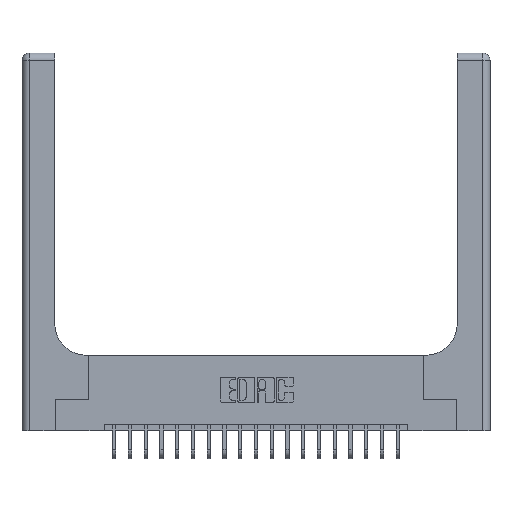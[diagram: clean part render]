
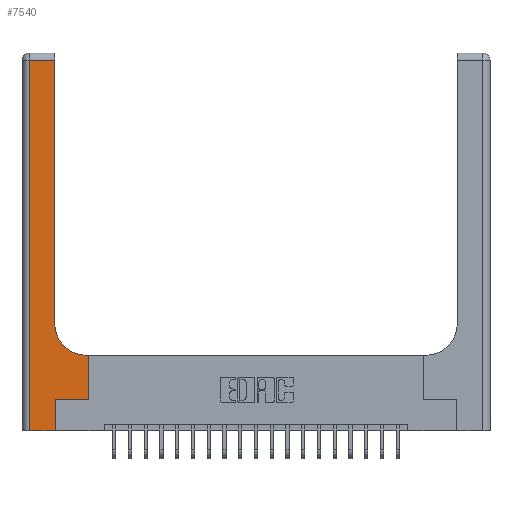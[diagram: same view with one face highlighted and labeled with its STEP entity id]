
A CAD part, top view. The second image highlights one B-rep face of the part: STEP entity #7540.
In plain terms, the highlighted planar face has unit normal (0, 0, 1).
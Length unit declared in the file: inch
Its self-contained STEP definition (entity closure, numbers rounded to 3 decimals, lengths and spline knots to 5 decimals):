
#25 = LINE ( 'NONE', #8723, #17636 ) ;
#267 = VERTEX_POINT ( 'NONE', #11001 ) ;
#465 = VERTEX_POINT ( 'NONE', #6812 ) ;
#708 = AXIS2_PLACEMENT_3D ( 'NONE', #6785, #1096, #18815 ) ;
#950 = DIRECTION ( 'NONE',  ( 0., 0., -1. ) ) ;
#1096 = DIRECTION ( 'NONE',  ( 0., 0., -1. ) ) ;
#1206 = VECTOR ( 'NONE', #18452, 39.37008 ) ;
#1271 = VERTEX_POINT ( 'NONE', #8339 ) ;
#1619 = EDGE_CURVE ( 'NONE', #19638, #19005, #4335, .T. ) ;
#1938 = ORIENTED_EDGE ( 'NONE', *, *, #16712, .T. ) ;
#2462 = CARTESIAN_POINT ( 'NONE',  ( 0.26, 2.94, 0.37 ) ) ;
#2492 = ORIENTED_EDGE ( 'NONE', *, *, #7852, .T. ) ;
#2962 = FACE_OUTER_BOUND ( 'NONE', #3066, .T. ) ;
#2971 = CARTESIAN_POINT ( 'NONE',  ( 0.26, 0.85, 0.37 ) ) ;
#3066 = EDGE_LOOP ( 'NONE', ( #18461, #1938, #12330, #13534, #17901, #19861, #5794, #11159, #2492 ) ) ;
#3070 = DIRECTION ( 'NONE',  ( -1., 0., 0. ) ) ;
#3158 = LINE ( 'NONE', #15536, #6835 ) ;
#3288 = DIRECTION ( 'NONE',  ( 0., -1., 0. ) ) ;
#3931 = VECTOR ( 'NONE', #7967, 39.37008 ) ;
#4335 = LINE ( 'NONE', #11410, #1206 ) ;
#4583 = EDGE_CURVE ( 'NONE', #13280, #6524, #16155, .T. ) ;
#4585 = PLANE ( 'NONE',  #708 ) ;
#5046 = CARTESIAN_POINT ( 'NONE',  ( 0., 2.94, 0.37 ) ) ;
#5384 = CARTESIAN_POINT ( 'NONE',  ( 0.528, 0.6, 0.37 ) ) ;
#5722 = VERTEX_POINT ( 'NONE', #7636 ) ;
#5794 = ORIENTED_EDGE ( 'NONE', *, *, #16874, .T. ) ;
#6521 = CARTESIAN_POINT ( 'NONE',  ( 0.51, 0.85, 0.37 ) ) ;
#6524 = VERTEX_POINT ( 'NONE', #2462 ) ;
#6785 = CARTESIAN_POINT ( 'NONE',  ( 0., 3., 0.37 ) ) ;
#6812 = CARTESIAN_POINT ( 'NONE',  ( 0.51, 0.6, 0.37 ) ) ;
#6835 = VECTOR ( 'NONE', #13585, 39.37008 ) ;
#7540 = ADVANCED_FACE ( 'NONE', ( #2962 ), #4585, .F. ) ;
#7636 = CARTESIAN_POINT ( 'NONE',  ( 0.06, 2.94, 0.37 ) ) ;
#7852 = EDGE_CURVE ( 'NONE', #465, #13280, #12595, .T. ) ;
#7967 = DIRECTION ( 'NONE',  ( 0., 1., 0. ) ) ;
#7998 = VECTOR ( 'NONE', #17659, 39.37008 ) ;
#8339 = CARTESIAN_POINT ( 'NONE',  ( 0.265, 0., 0.37 ) ) ;
#8443 = LINE ( 'NONE', #13892, #21666 ) ;
#8723 = CARTESIAN_POINT ( 'NONE',  ( 0.06, 3., 0.37 ) ) ;
#9207 = VECTOR ( 'NONE', #21513, 39.37008 ) ;
#10215 = CARTESIAN_POINT ( 'NONE',  ( 0.528, 0.25, 0.37 ) ) ;
#10853 = CARTESIAN_POINT ( 'NONE',  ( 0.26, 3., 0.37 ) ) ;
#11001 = CARTESIAN_POINT ( 'NONE',  ( 0.06, 0., 0.37 ) ) ;
#11159 = ORIENTED_EDGE ( 'NONE', *, *, #13046, .T. ) ;
#11332 = VECTOR ( 'NONE', #3070, 39.37008 ) ;
#11410 = CARTESIAN_POINT ( 'NONE',  ( 0.265, 0.25, 0.37 ) ) ;
#12330 = ORIENTED_EDGE ( 'NONE', *, *, #21601, .T. ) ;
#12595 = CIRCLE ( 'NONE', #18850, 0.25 ) ;
#13046 = EDGE_CURVE ( 'NONE', #18765, #465, #3158, .T. ) ;
#13280 = VERTEX_POINT ( 'NONE', #2971 ) ;
#13534 = ORIENTED_EDGE ( 'NONE', *, *, #18340, .T. ) ;
#13585 = DIRECTION ( 'NONE',  ( -1., 0., 0. ) ) ;
#13892 = CARTESIAN_POINT ( 'NONE',  ( 0., 0., 0.37 ) ) ;
#15447 = LINE ( 'NONE', #5046, #11332 ) ;
#15536 = CARTESIAN_POINT ( 'NONE',  ( 0.26, 0.6, 0.37 ) ) ;
#16155 = LINE ( 'NONE', #10853, #9207 ) ;
#16712 = EDGE_CURVE ( 'NONE', #6524, #5722, #15447, .T. ) ;
#16874 = EDGE_CURVE ( 'NONE', #19005, #18765, #21492, .T. ) ;
#16933 = DIRECTION ( 'NONE',  ( 1., 0., 0. ) ) ;
#17636 = VECTOR ( 'NONE', #3288, 39.37008 ) ;
#17659 = DIRECTION ( 'NONE',  ( 0., 1., 0. ) ) ;
#17901 = ORIENTED_EDGE ( 'NONE', *, *, #21127, .T. ) ;
#18340 = EDGE_CURVE ( 'NONE', #267, #1271, #8443, .T. ) ;
#18452 = DIRECTION ( 'NONE',  ( 1., 0., 0. ) ) ;
#18461 = ORIENTED_EDGE ( 'NONE', *, *, #4583, .T. ) ;
#18765 = VERTEX_POINT ( 'NONE', #5384 ) ;
#18815 = DIRECTION ( 'NONE',  ( -1., 0., 0. ) ) ;
#18850 = AXIS2_PLACEMENT_3D ( 'NONE', #6521, #950, #16933 ) ;
#18956 = LINE ( 'NONE', #22105, #3931 ) ;
#19005 = VERTEX_POINT ( 'NONE', #10215 ) ;
#19638 = VERTEX_POINT ( 'NONE', #21880 ) ;
#19861 = ORIENTED_EDGE ( 'NONE', *, *, #1619, .T. ) ;
#20167 = CARTESIAN_POINT ( 'NONE',  ( 0.528, 0.25, 0.37 ) ) ;
#21082 = DIRECTION ( 'NONE',  ( 1., 0., 0. ) ) ;
#21127 = EDGE_CURVE ( 'NONE', #1271, #19638, #18956, .T. ) ;
#21492 = LINE ( 'NONE', #20167, #7998 ) ;
#21513 = DIRECTION ( 'NONE',  ( 0., 1., 0. ) ) ;
#21601 = EDGE_CURVE ( 'NONE', #5722, #267, #25, .T. ) ;
#21666 = VECTOR ( 'NONE', #21082, 39.37008 ) ;
#21880 = CARTESIAN_POINT ( 'NONE',  ( 0.265, 0.25, 0.37 ) ) ;
#22105 = CARTESIAN_POINT ( 'NONE',  ( 0.265, 0., 0.37 ) ) ;
